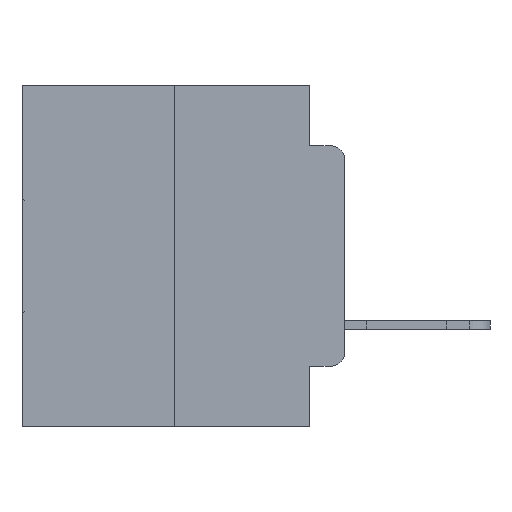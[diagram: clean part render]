
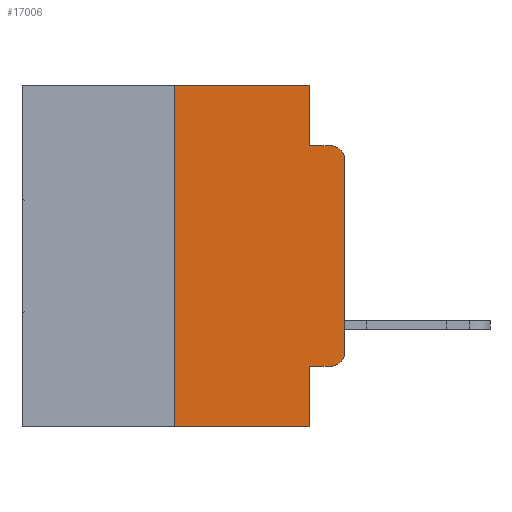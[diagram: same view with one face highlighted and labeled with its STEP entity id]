
A CAD part, left-side view. The second image highlights one B-rep face of the part: STEP entity #17006.
In plain terms, the highlighted planar face has unit normal (-1, 0, 0).
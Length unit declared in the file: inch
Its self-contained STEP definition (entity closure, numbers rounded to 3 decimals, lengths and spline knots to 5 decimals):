
#1039 = EDGE_CURVE ( 'NONE', #25310, #20471, #18039, .T. ) ;
#1494 = VERTEX_POINT ( 'NONE', #24517 ) ;
#1866 = CARTESIAN_POINT ( 'NONE',  ( 0., 0.473, 0. ) ) ;
#1924 = ORIENTED_EDGE ( 'NONE', *, *, #21951, .F. ) ;
#1962 = DIRECTION ( 'NONE',  ( 1., 0., 0. ) ) ;
#2262 = VERTEX_POINT ( 'NONE', #6941 ) ;
#2440 = EDGE_CURVE ( 'NONE', #2735, #28669, #23806, .T. ) ;
#2484 = EDGE_LOOP ( 'NONE', ( #13090, #23029, #7041, #10255, #1924, #3082, #2993, #20784, #21167, #27188 ) ) ;
#2569 = CARTESIAN_POINT ( 'NONE',  ( 0., 0.051, 0. ) ) ;
#2735 = VERTEX_POINT ( 'NONE', #23383 ) ;
#2993 = ORIENTED_EDGE ( 'NONE', *, *, #18492, .T. ) ;
#3012 = CARTESIAN_POINT ( 'NONE',  ( 0., 0., -0.3915 ) ) ;
#3082 = ORIENTED_EDGE ( 'NONE', *, *, #12034, .F. ) ;
#3368 = CARTESIAN_POINT ( 'NONE',  ( 0., 0.473, 0. ) ) ;
#4870 = CARTESIAN_POINT ( 'NONE',  ( 0., 0.02, -0.1085 ) ) ;
#4994 = CARTESIAN_POINT ( 'NONE',  ( 0., 0.051, -0.4115 ) ) ;
#6415 = DIRECTION ( 'NONE',  ( 0., 0., -1. ) ) ;
#6941 = CARTESIAN_POINT ( 'NONE',  ( 0., 0.051, -0.5 ) ) ;
#6955 = EDGE_CURVE ( 'NONE', #17045, #28669, #9378, .T. ) ;
#7041 = ORIENTED_EDGE ( 'NONE', *, *, #6955, .F. ) ;
#7344 = DIRECTION ( 'NONE',  ( 0., 0., -1. ) ) ;
#7367 = DIRECTION ( 'NONE',  ( 0., -1., 0. ) ) ;
#7608 = CARTESIAN_POINT ( 'NONE',  ( 0., 0.02, -0.4115 ) ) ;
#7838 = EDGE_CURVE ( 'NONE', #21818, #17045, #8562, .T. ) ;
#8562 = LINE ( 'NONE', #20510, #22586 ) ;
#8725 = CARTESIAN_POINT ( 'NONE',  ( 0., 0.25, -0.5 ) ) ;
#8828 = DIRECTION ( 'NONE',  ( 0., 0., 1. ) ) ;
#8892 = CARTESIAN_POINT ( 'NONE',  ( 0., 0.02, -0.3915 ) ) ;
#9001 = DIRECTION ( 'NONE',  ( 0., 0., -1. ) ) ;
#9019 = VECTOR ( 'NONE', #7367, 39.37008 ) ;
#9058 = CARTESIAN_POINT ( 'NONE',  ( 0., 0.051, -0.4115 ) ) ;
#9378 = LINE ( 'NONE', #14497, #9019 ) ;
#9961 = EDGE_CURVE ( 'NONE', #16563, #25310, #17299, .T. ) ;
#10019 = CARTESIAN_POINT ( 'NONE',  ( 0., 0.051, 0. ) ) ;
#10255 = ORIENTED_EDGE ( 'NONE', *, *, #7838, .F. ) ;
#10274 = DIRECTION ( 'NONE',  ( 0., 0., 1. ) ) ;
#11444 = DIRECTION ( 'NONE',  ( 0., -1., 0. ) ) ;
#11498 = DIRECTION ( 'NONE',  ( -1., 0., 0. ) ) ;
#11675 = LINE ( 'NONE', #27616, #28965 ) ;
#12034 = EDGE_CURVE ( 'NONE', #17204, #1494, #14586, .T. ) ;
#13090 = ORIENTED_EDGE ( 'NONE', *, *, #19021, .T. ) ;
#13278 = CARTESIAN_POINT ( 'NONE',  ( 0., 0.25, 0. ) ) ;
#13468 = DIRECTION ( 'NONE',  ( 0., -1., 0. ) ) ;
#14497 = CARTESIAN_POINT ( 'NONE',  ( 0., 0.051, -0.0885 ) ) ;
#14586 = LINE ( 'NONE', #13278, #29004 ) ;
#14657 = CARTESIAN_POINT ( 'NONE',  ( 0., 0.02, -0.0885 ) ) ;
#14664 = FACE_OUTER_BOUND ( 'NONE', #2484, .T. ) ;
#14904 = LINE ( 'NONE', #3368, #15309 ) ;
#15023 = AXIS2_PLACEMENT_3D ( 'NONE', #8892, #11498, #9001 ) ;
#15309 = VECTOR ( 'NONE', #24952, 39.37008 ) ;
#16563 = VERTEX_POINT ( 'NONE', #4994 ) ;
#16593 = VECTOR ( 'NONE', #11444, 39.37008 ) ;
#16790 = DIRECTION ( 'NONE',  ( -1., 0., 0. ) ) ;
#17006 = ADVANCED_FACE ( 'NONE', ( #14664 ), #25626, .F. ) ;
#17045 = VERTEX_POINT ( 'NONE', #30258 ) ;
#17204 = VERTEX_POINT ( 'NONE', #8725 ) ;
#17299 = LINE ( 'NONE', #9058, #16593 ) ;
#18039 = CIRCLE ( 'NONE', #15023, 0.02 ) ;
#18042 = DIRECTION ( 'NONE',  ( 0., 0., -1. ) ) ;
#18425 = LINE ( 'NONE', #29962, #23906 ) ;
#18492 = EDGE_CURVE ( 'NONE', #17204, #2262, #11675, .T. ) ;
#19021 = EDGE_CURVE ( 'NONE', #20471, #2735, #18425, .T. ) ;
#20368 = DIRECTION ( 'NONE',  ( 0., 0., -1. ) ) ;
#20421 = AXIS2_PLACEMENT_3D ( 'NONE', #4870, #16790, #7344 ) ;
#20471 = VERTEX_POINT ( 'NONE', #3012 ) ;
#20510 = CARTESIAN_POINT ( 'NONE',  ( 0., 0.051, 0. ) ) ;
#20784 = ORIENTED_EDGE ( 'NONE', *, *, #24761, .F. ) ;
#21167 = ORIENTED_EDGE ( 'NONE', *, *, #9961, .T. ) ;
#21732 = VECTOR ( 'NONE', #20368, 39.37008 ) ;
#21818 = VERTEX_POINT ( 'NONE', #10019 ) ;
#21951 = EDGE_CURVE ( 'NONE', #1494, #21818, #14904, .T. ) ;
#22483 = AXIS2_PLACEMENT_3D ( 'NONE', #1866, #1962, #6415 ) ;
#22586 = VECTOR ( 'NONE', #18042, 39.37008 ) ;
#23029 = ORIENTED_EDGE ( 'NONE', *, *, #2440, .T. ) ;
#23383 = CARTESIAN_POINT ( 'NONE',  ( 0., 0., -0.1085 ) ) ;
#23806 = CIRCLE ( 'NONE', #20421, 0.02 ) ;
#23906 = VECTOR ( 'NONE', #8828, 39.37008 ) ;
#24517 = CARTESIAN_POINT ( 'NONE',  ( 0., 0.25, 0. ) ) ;
#24761 = EDGE_CURVE ( 'NONE', #16563, #2262, #29510, .T. ) ;
#24952 = DIRECTION ( 'NONE',  ( 0., -1., 0. ) ) ;
#25310 = VERTEX_POINT ( 'NONE', #7608 ) ;
#25626 = PLANE ( 'NONE',  #22483 ) ;
#27188 = ORIENTED_EDGE ( 'NONE', *, *, #1039, .T. ) ;
#27616 = CARTESIAN_POINT ( 'NONE',  ( 0., 0.473, -0.5 ) ) ;
#28669 = VERTEX_POINT ( 'NONE', #14657 ) ;
#28965 = VECTOR ( 'NONE', #13468, 39.37008 ) ;
#29004 = VECTOR ( 'NONE', #10274, 39.37008 ) ;
#29510 = LINE ( 'NONE', #2569, #21732 ) ;
#29962 = CARTESIAN_POINT ( 'NONE',  ( 0., 0., 0. ) ) ;
#30258 = CARTESIAN_POINT ( 'NONE',  ( 0., 0.051, -0.0885 ) ) ;
